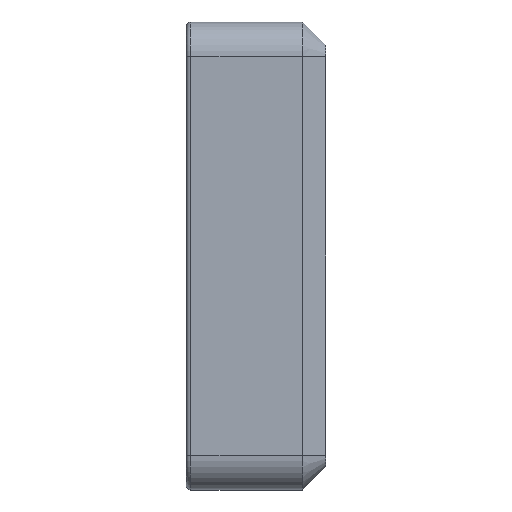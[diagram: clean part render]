
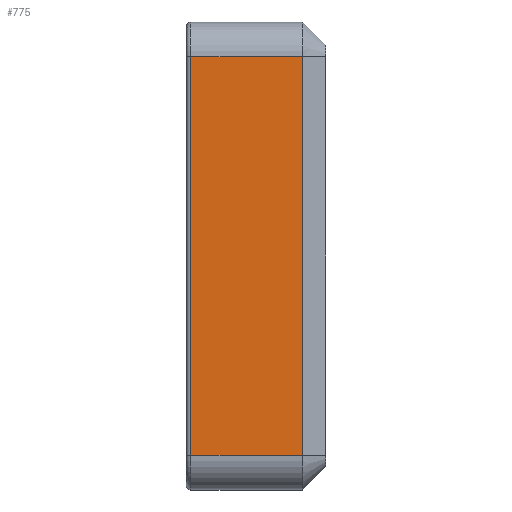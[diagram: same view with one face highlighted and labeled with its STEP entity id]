
A CAD part, front view. The second image highlights one B-rep face of the part: STEP entity #775.
In plain terms, the highlighted planar face has unit normal (0, -1, 0).
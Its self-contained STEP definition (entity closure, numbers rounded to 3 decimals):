
#18 = DIRECTION ( 'NONE',  ( -1., 0., 0. ) ) ;
#35 = VERTEX_POINT ( 'NONE', #262 ) ;
#45 = EDGE_CURVE ( 'NONE', #319, #708, #558, .T. ) ;
#74 = ORIENTED_EDGE ( 'NONE', *, *, #1478, .F. ) ;
#120 = CARTESIAN_POINT ( 'NONE',  ( 106.718, 0.06, -17.1 ) ) ;
#168 = ORIENTED_EDGE ( 'NONE', *, *, #930, .F. ) ;
#198 = CARTESIAN_POINT ( 'NONE',  ( 113.566, 0.06, 18.535 ) ) ;
#207 = CARTESIAN_POINT ( 'NONE',  ( 116.318, 0.06, 10.631 ) ) ;
#218 = DIRECTION ( 'NONE',  ( 0., 0., -1. ) ) ;
#262 = CARTESIAN_POINT ( 'NONE',  ( 116.318, 0.06, -17.1 ) ) ;
#311 = DIRECTION ( 'NONE',  ( 0., 0., -1. ) ) ;
#319 = VERTEX_POINT ( 'NONE', #777 ) ;
#344 = LINE ( 'NONE', #207, #1150 ) ;
#400 = ORIENTED_EDGE ( 'NONE', *, *, #45, .F. ) ;
#428 = VERTEX_POINT ( 'NONE', #120 ) ;
#469 = LINE ( 'NONE', #1180, #691 ) ;
#539 = DIRECTION ( 'NONE',  ( 0., 0., 1. ) ) ;
#558 = LINE ( 'NONE', #845, #1249 ) ;
#658 = PLANE ( 'NONE',  #821 ) ;
#666 = LINE ( 'NONE', #898, #1342 ) ;
#691 = VECTOR ( 'NONE', #18, 1000. ) ;
#708 = VERTEX_POINT ( 'NONE', #992 ) ;
#775 = ADVANCED_FACE ( 'NONE', ( #1353 ), #658, .T. ) ;
#777 = CARTESIAN_POINT ( 'NONE',  ( 106.718, 0.06, 17.1 ) ) ;
#781 = DIRECTION ( 'NONE',  ( 0., -1., 0. ) ) ;
#821 = AXIS2_PLACEMENT_3D ( 'NONE', #198, #781, #311 ) ;
#845 = CARTESIAN_POINT ( 'NONE',  ( 113.566, 0.06, 17.1 ) ) ;
#875 = EDGE_CURVE ( 'NONE', #428, #319, #666, .T. ) ;
#898 = CARTESIAN_POINT ( 'NONE',  ( 106.718, 0.06, 9.268 ) ) ;
#930 = EDGE_CURVE ( 'NONE', #708, #35, #344, .T. ) ;
#992 = CARTESIAN_POINT ( 'NONE',  ( 116.318, 0.06, 17.1 ) ) ;
#1016 = EDGE_LOOP ( 'NONE', ( #1322, #74, #168, #400 ) ) ;
#1081 = DIRECTION ( 'NONE',  ( 1., 0., 0. ) ) ;
#1150 = VECTOR ( 'NONE', #218, 1000. ) ;
#1180 = CARTESIAN_POINT ( 'NONE',  ( 114.782, 0.06, -17.1 ) ) ;
#1249 = VECTOR ( 'NONE', #1081, 1000. ) ;
#1322 = ORIENTED_EDGE ( 'NONE', *, *, #875, .F. ) ;
#1342 = VECTOR ( 'NONE', #539, 1000. ) ;
#1353 = FACE_OUTER_BOUND ( 'NONE', #1016, .T. ) ;
#1478 = EDGE_CURVE ( 'NONE', #35, #428, #469, .T. ) ;
